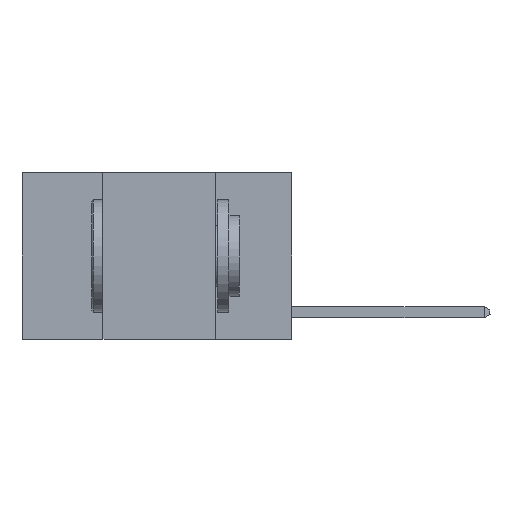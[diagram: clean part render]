
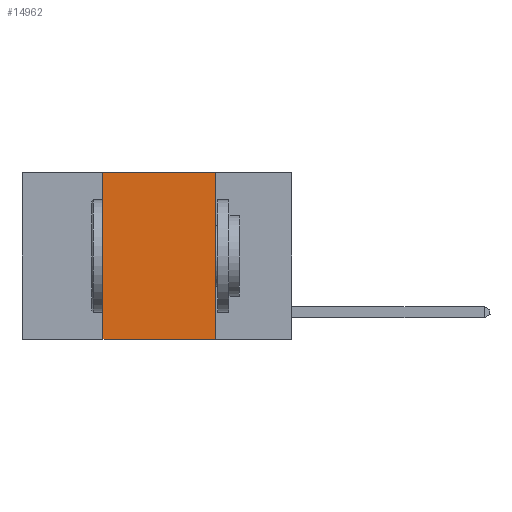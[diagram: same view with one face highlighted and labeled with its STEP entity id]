
A CAD part, left-side view. The second image highlights one B-rep face of the part: STEP entity #14962.
In plain terms, the highlighted planar face has unit normal (-1, 0, 0).
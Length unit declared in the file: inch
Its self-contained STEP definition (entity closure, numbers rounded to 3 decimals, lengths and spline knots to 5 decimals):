
#1428 = DIRECTION ( 'NONE',  ( 0., 0., -1. ) ) ;
#1598 = DIRECTION ( 'NONE',  ( 0., -1., 0. ) ) ;
#2211 = VECTOR ( 'NONE', #5771, 39.37008 ) ;
#2391 = VERTEX_POINT ( 'NONE', #23300 ) ;
#2401 = CARTESIAN_POINT ( 'NONE',  ( 0., 0.17, 0. ) ) ;
#2934 = EDGE_CURVE ( 'NONE', #10016, #23932, #21322, .T. ) ;
#3475 = CARTESIAN_POINT ( 'NONE',  ( 0., 0.6, 0. ) ) ;
#4219 = DIRECTION ( 'NONE',  ( 0., 0., 1. ) ) ;
#5137 = ORIENTED_EDGE ( 'NONE', *, *, #23404, .F. ) ;
#5771 = DIRECTION ( 'NONE',  ( 0., -1., 0. ) ) ;
#7359 = DIRECTION ( 'NONE',  ( 0., 0., -1. ) ) ;
#8053 = ORIENTED_EDGE ( 'NONE', *, *, #2934, .F. ) ;
#8703 = CARTESIAN_POINT ( 'NONE',  ( 0., 0.42, -0.37 ) ) ;
#8740 = CARTESIAN_POINT ( 'NONE',  ( 0., 0.17, -0.37 ) ) ;
#10016 = VERTEX_POINT ( 'NONE', #23037 ) ;
#10625 = VECTOR ( 'NONE', #4219, 39.37008 ) ;
#10843 = VECTOR ( 'NONE', #1598, 39.37008 ) ;
#11932 = DIRECTION ( 'NONE',  ( 1., 0., 0. ) ) ;
#12394 = CARTESIAN_POINT ( 'NONE',  ( 0., 0.42, 0. ) ) ;
#13686 = ORIENTED_EDGE ( 'NONE', *, *, #20654, .F. ) ;
#14008 = PLANE ( 'NONE',  #15665 ) ;
#14489 = CARTESIAN_POINT ( 'NONE',  ( 0., 0.6, 0. ) ) ;
#14496 = EDGE_CURVE ( 'NONE', #23110, #23932, #22032, .T. ) ;
#14962 = ADVANCED_FACE ( 'NONE', ( #22410 ), #14008, .F. ) ;
#15665 = AXIS2_PLACEMENT_3D ( 'NONE', #3475, #11932, #1428 ) ;
#15842 = CARTESIAN_POINT ( 'NONE',  ( 0., 0.6, -0.37 ) ) ;
#16159 = LINE ( 'NONE', #14489, #2211 ) ;
#20654 = EDGE_CURVE ( 'NONE', #2391, #10016, #16159, .T. ) ;
#20758 = EDGE_LOOP ( 'NONE', ( #8053, #13686, #5137, #24900 ) ) ;
#20942 = VECTOR ( 'NONE', #7359, 39.37008 ) ;
#21322 = LINE ( 'NONE', #2401, #20942 ) ;
#22032 = LINE ( 'NONE', #15842, #10843 ) ;
#22410 = FACE_OUTER_BOUND ( 'NONE', #20758, .T. ) ;
#23037 = CARTESIAN_POINT ( 'NONE',  ( 0., 0.17, 0. ) ) ;
#23110 = VERTEX_POINT ( 'NONE', #8703 ) ;
#23154 = LINE ( 'NONE', #12394, #10625 ) ;
#23300 = CARTESIAN_POINT ( 'NONE',  ( 0., 0.42, 0. ) ) ;
#23404 = EDGE_CURVE ( 'NONE', #23110, #2391, #23154, .T. ) ;
#23932 = VERTEX_POINT ( 'NONE', #8740 ) ;
#24900 = ORIENTED_EDGE ( 'NONE', *, *, #14496, .T. ) ;
